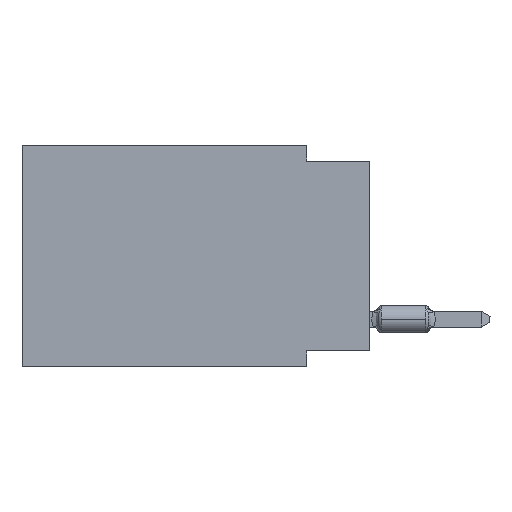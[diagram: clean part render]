
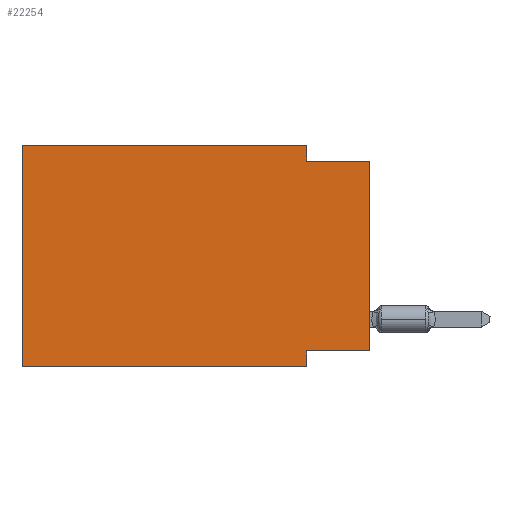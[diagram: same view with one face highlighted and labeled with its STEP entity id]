
A CAD part, left-side view. The second image highlights one B-rep face of the part: STEP entity #22254.
In plain terms, the highlighted planar face has unit normal (-1, 0, 0).
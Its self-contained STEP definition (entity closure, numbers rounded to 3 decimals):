
#507 = LINE ( 'NONE', #17358, #3155 ) ;
#616 = CARTESIAN_POINT ( 'NONE',  ( 0., 0., -0.635 ) ) ;
#806 = AXIS2_PLACEMENT_3D ( 'NONE', #3586, #19384, #25505 ) ;
#1360 = VERTEX_POINT ( 'NONE', #15090 ) ;
#3033 = ORIENTED_EDGE ( 'NONE', *, *, #26652, .F. ) ;
#3155 = VECTOR ( 'NONE', #38242, 1000. ) ;
#3586 = CARTESIAN_POINT ( 'NONE',  ( 0., 13.97, 0. ) ) ;
#3998 = EDGE_CURVE ( 'NONE', #24290, #20060, #46593, .T. ) ;
#5638 = LINE ( 'NONE', #10449, #36015 ) ;
#5754 = DIRECTION ( 'NONE',  ( 0., -1., 0. ) ) ;
#6057 = VECTOR ( 'NONE', #45095, 1000. ) ;
#6124 = DIRECTION ( 'NONE',  ( 0., -1., 0. ) ) ;
#6397 = LINE ( 'NONE', #8084, #22372 ) ;
#6632 = EDGE_CURVE ( 'NONE', #16893, #16026, #51235, .T. ) ;
#7899 = CARTESIAN_POINT ( 'NONE',  ( 0., 2.54, -8.89 ) ) ;
#8084 = CARTESIAN_POINT ( 'NONE',  ( 0., 13.97, 0. ) ) ;
#8276 = CARTESIAN_POINT ( 'NONE',  ( 0., 2.54, 0. ) ) ;
#8431 = LINE ( 'NONE', #50905, #6057 ) ;
#9765 = DIRECTION ( 'NONE',  ( 0., 1., 0. ) ) ;
#10117 = DIRECTION ( 'NONE',  ( 0., 0., 1. ) ) ;
#10449 = CARTESIAN_POINT ( 'NONE',  ( 0., 0., 0. ) ) ;
#12278 = CARTESIAN_POINT ( 'NONE',  ( 0., 13.97, -8.89 ) ) ;
#14021 = ORIENTED_EDGE ( 'NONE', *, *, #18435, .F. ) ;
#14300 = CARTESIAN_POINT ( 'NONE',  ( 0., 2.54, -0.635 ) ) ;
#15090 = CARTESIAN_POINT ( 'NONE',  ( 0., 13.97, 0. ) ) ;
#16026 = VERTEX_POINT ( 'NONE', #49531 ) ;
#16893 = VERTEX_POINT ( 'NONE', #50787 ) ;
#17358 = CARTESIAN_POINT ( 'NONE',  ( 0., 2.54, 0. ) ) ;
#17810 = CARTESIAN_POINT ( 'NONE',  ( 0., 2.54, -8.89 ) ) ;
#18435 = EDGE_CURVE ( 'NONE', #16026, #47535, #28811, .T. ) ;
#18504 = ORIENTED_EDGE ( 'NONE', *, *, #41132, .F. ) ;
#19384 = DIRECTION ( 'NONE',  ( 1., 0., 0. ) ) ;
#20060 = VERTEX_POINT ( 'NONE', #26111 ) ;
#22254 = ADVANCED_FACE ( 'NONE', ( #60836 ), #50545, .F. ) ;
#22372 = VECTOR ( 'NONE', #49549, 1000. ) ;
#24290 = VERTEX_POINT ( 'NONE', #14300 ) ;
#25505 = DIRECTION ( 'NONE',  ( 0., 0., -1. ) ) ;
#25513 = VECTOR ( 'NONE', #6124, 1000. ) ;
#26111 = CARTESIAN_POINT ( 'NONE',  ( 0., 0., -0.635 ) ) ;
#26213 = EDGE_LOOP ( 'NONE', ( #41243, #39751, #18504, #3033, #41571, #27418, #14021, #31273 ) ) ;
#26652 = EDGE_CURVE ( 'NONE', #1360, #47194, #8431, .T. ) ;
#27418 = ORIENTED_EDGE ( 'NONE', *, *, #34726, .T. ) ;
#28486 = VECTOR ( 'NONE', #9765, 1000. ) ;
#28811 = LINE ( 'NONE', #7899, #64325 ) ;
#31273 = ORIENTED_EDGE ( 'NONE', *, *, #6632, .F. ) ;
#31617 = VERTEX_POINT ( 'NONE', #12278 ) ;
#32499 = LINE ( 'NONE', #53405, #44615 ) ;
#34726 = EDGE_CURVE ( 'NONE', #31617, #47535, #32499, .T. ) ;
#35808 = CARTESIAN_POINT ( 'NONE',  ( 0., 0., -8.255 ) ) ;
#36015 = VECTOR ( 'NONE', #10117, 1000. ) ;
#38093 = EDGE_CURVE ( 'NONE', #16893, #20060, #5638, .T. ) ;
#38242 = DIRECTION ( 'NONE',  ( 0., 0., -1. ) ) ;
#39751 = ORIENTED_EDGE ( 'NONE', *, *, #3998, .F. ) ;
#41132 = EDGE_CURVE ( 'NONE', #47194, #24290, #507, .T. ) ;
#41243 = ORIENTED_EDGE ( 'NONE', *, *, #38093, .T. ) ;
#41571 = ORIENTED_EDGE ( 'NONE', *, *, #61349, .F. ) ;
#44615 = VECTOR ( 'NONE', #5754, 1000. ) ;
#45095 = DIRECTION ( 'NONE',  ( 0., -1., 0. ) ) ;
#46593 = LINE ( 'NONE', #616, #25513 ) ;
#47194 = VERTEX_POINT ( 'NONE', #8276 ) ;
#47535 = VERTEX_POINT ( 'NONE', #17810 ) ;
#49531 = CARTESIAN_POINT ( 'NONE',  ( 0., 2.54, -8.255 ) ) ;
#49549 = DIRECTION ( 'NONE',  ( 0., 0., 1. ) ) ;
#50383 = DIRECTION ( 'NONE',  ( 0., 0., -1. ) ) ;
#50545 = PLANE ( 'NONE',  #806 ) ;
#50787 = CARTESIAN_POINT ( 'NONE',  ( 0., 0., -8.255 ) ) ;
#50905 = CARTESIAN_POINT ( 'NONE',  ( 0., 13.97, 0. ) ) ;
#51235 = LINE ( 'NONE', #35808, #28486 ) ;
#53405 = CARTESIAN_POINT ( 'NONE',  ( 0., 13.97, -8.89 ) ) ;
#60836 = FACE_OUTER_BOUND ( 'NONE', #26213, .T. ) ;
#61349 = EDGE_CURVE ( 'NONE', #31617, #1360, #6397, .T. ) ;
#64325 = VECTOR ( 'NONE', #50383, 1000. ) ;
